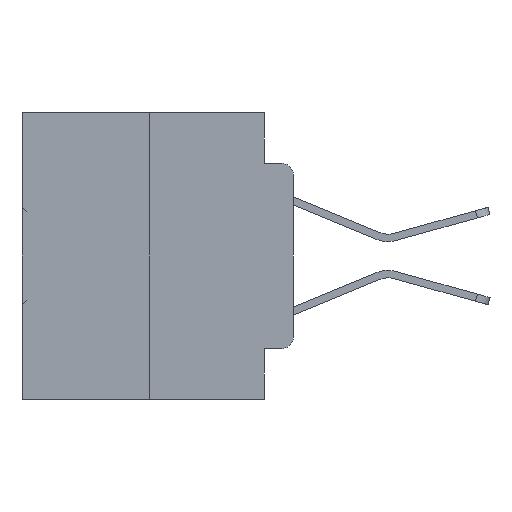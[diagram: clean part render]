
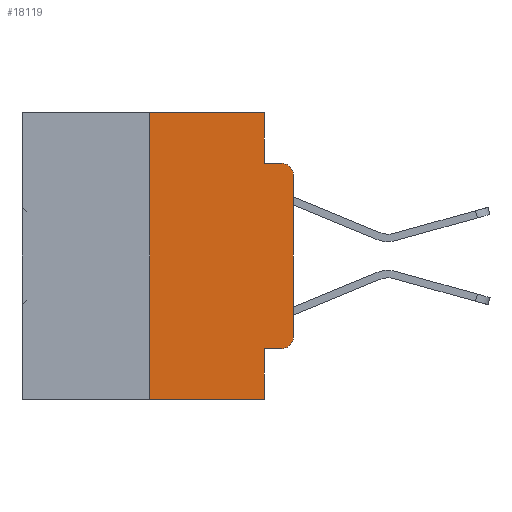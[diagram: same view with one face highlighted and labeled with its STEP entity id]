
A CAD part, left-side view. The second image highlights one B-rep face of the part: STEP entity #18119.
In plain terms, the highlighted planar face has unit normal (-1, 0, 0).
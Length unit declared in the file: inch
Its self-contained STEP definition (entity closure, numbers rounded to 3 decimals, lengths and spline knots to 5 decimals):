
#815 = CARTESIAN_POINT ( 'NONE',  ( 0., 0.02, -0.1085 ) ) ;
#1361 = VECTOR ( 'NONE', #24522, 39.37008 ) ;
#1391 = VERTEX_POINT ( 'NONE', #7197 ) ;
#2439 = VECTOR ( 'NONE', #12109, 39.37008 ) ;
#3083 = CARTESIAN_POINT ( 'NONE',  ( 0., 0.473, 0. ) ) ;
#3580 = DIRECTION ( 'NONE',  ( -1., 0., 0. ) ) ;
#4086 = CARTESIAN_POINT ( 'NONE',  ( 0., 0.02, -0.4115 ) ) ;
#4298 = DIRECTION ( 'NONE',  ( 0., 0., -1. ) ) ;
#4858 = ORIENTED_EDGE ( 'NONE', *, *, #23717, .F. ) ;
#5162 = VECTOR ( 'NONE', #30448, 39.37008 ) ;
#5226 = EDGE_CURVE ( 'NONE', #23776, #33122, #32588, .T. ) ;
#5251 = DIRECTION ( 'NONE',  ( 0., 0., -1. ) ) ;
#5301 = CARTESIAN_POINT ( 'NONE',  ( 0., 0.473, 0. ) ) ;
#6832 = CARTESIAN_POINT ( 'NONE',  ( 0., 0., -0.1085 ) ) ;
#7024 = CARTESIAN_POINT ( 'NONE',  ( 0., 0.051, 0. ) ) ;
#7197 = CARTESIAN_POINT ( 'NONE',  ( 0., 0.02, -0.0885 ) ) ;
#7627 = VERTEX_POINT ( 'NONE', #16283 ) ;
#8109 = VECTOR ( 'NONE', #4298, 39.37008 ) ;
#8132 = LINE ( 'NONE', #9540, #15769 ) ;
#8740 = DIRECTION ( 'NONE',  ( 0., 0., -1. ) ) ;
#9258 = FACE_OUTER_BOUND ( 'NONE', #24429, .T. ) ;
#9540 = CARTESIAN_POINT ( 'NONE',  ( 0., 0.051, -0.0885 ) ) ;
#9782 = CARTESIAN_POINT ( 'NONE',  ( 0., 0.051, -0.0885 ) ) ;
#9805 = VERTEX_POINT ( 'NONE', #14158 ) ;
#10071 = VECTOR ( 'NONE', #30102, 39.37008 ) ;
#10455 = LINE ( 'NONE', #14691, #2439 ) ;
#11092 = CARTESIAN_POINT ( 'NONE',  ( 0., 0.051, -0.4115 ) ) ;
#11352 = EDGE_CURVE ( 'NONE', #15332, #1391, #22079, .T. ) ;
#11834 = LINE ( 'NONE', #3083, #5162 ) ;
#12075 = CARTESIAN_POINT ( 'NONE',  ( 0., 0., 0. ) ) ;
#12109 = DIRECTION ( 'NONE',  ( 0., 0., 1. ) ) ;
#12457 = LINE ( 'NONE', #7024, #23057 ) ;
#13228 = ORIENTED_EDGE ( 'NONE', *, *, #14233, .F. ) ;
#13718 = EDGE_CURVE ( 'NONE', #17415, #15332, #17701, .T. ) ;
#13754 = AXIS2_PLACEMENT_3D ( 'NONE', #26885, #19179, #5251 ) ;
#14158 = CARTESIAN_POINT ( 'NONE',  ( 0., 0.051, -0.5 ) ) ;
#14233 = EDGE_CURVE ( 'NONE', #23814, #7627, #10455, .T. ) ;
#14691 = CARTESIAN_POINT ( 'NONE',  ( 0., 0.25, 0. ) ) ;
#15332 = VERTEX_POINT ( 'NONE', #6832 ) ;
#15384 = AXIS2_PLACEMENT_3D ( 'NONE', #5301, #26608, #24231 ) ;
#15484 = ORIENTED_EDGE ( 'NONE', *, *, #24809, .F. ) ;
#15769 = VECTOR ( 'NONE', #31266, 39.37008 ) ;
#15909 = PLANE ( 'NONE',  #15384 ) ;
#16283 = CARTESIAN_POINT ( 'NONE',  ( 0., 0.25, 0. ) ) ;
#16669 = EDGE_CURVE ( 'NONE', #22146, #18625, #17399, .T. ) ;
#17399 = LINE ( 'NONE', #33327, #8109 ) ;
#17415 = VERTEX_POINT ( 'NONE', #24233 ) ;
#17701 = LINE ( 'NONE', #12075, #18967 ) ;
#18119 = ADVANCED_FACE ( 'NONE', ( #9258 ), #15909, .F. ) ;
#18625 = VERTEX_POINT ( 'NONE', #9782 ) ;
#18967 = VECTOR ( 'NONE', #34099, 39.37008 ) ;
#19179 = DIRECTION ( 'NONE',  ( -1., 0., 0. ) ) ;
#20982 = DIRECTION ( 'NONE',  ( 0., 0., -1. ) ) ;
#21696 = ORIENTED_EDGE ( 'NONE', *, *, #13718, .T. ) ;
#22061 = ORIENTED_EDGE ( 'NONE', *, *, #5226, .T. ) ;
#22079 = CIRCLE ( 'NONE', #35113, 0.02 ) ;
#22146 = VERTEX_POINT ( 'NONE', #26812 ) ;
#22573 = EDGE_CURVE ( 'NONE', #23776, #9805, #12457, .T. ) ;
#22781 = CARTESIAN_POINT ( 'NONE',  ( 0., 0.25, -0.5 ) ) ;
#23057 = VECTOR ( 'NONE', #20982, 39.37008 ) ;
#23717 = EDGE_CURVE ( 'NONE', #18625, #1391, #8132, .T. ) ;
#23776 = VERTEX_POINT ( 'NONE', #33778 ) ;
#23814 = VERTEX_POINT ( 'NONE', #22781 ) ;
#24160 = EDGE_CURVE ( 'NONE', #23814, #9805, #25488, .T. ) ;
#24231 = DIRECTION ( 'NONE',  ( 0., 0., -1. ) ) ;
#24233 = CARTESIAN_POINT ( 'NONE',  ( 0., 0., -0.3915 ) ) ;
#24429 = EDGE_LOOP ( 'NONE', ( #21696, #26432, #4858, #33226, #15484, #13228, #32998, #26141, #22061, #33132 ) ) ;
#24522 = DIRECTION ( 'NONE',  ( 0., -1., 0. ) ) ;
#24809 = EDGE_CURVE ( 'NONE', #7627, #22146, #11834, .T. ) ;
#25488 = LINE ( 'NONE', #30372, #1361 ) ;
#26141 = ORIENTED_EDGE ( 'NONE', *, *, #22573, .F. ) ;
#26432 = ORIENTED_EDGE ( 'NONE', *, *, #11352, .T. ) ;
#26608 = DIRECTION ( 'NONE',  ( 1., 0., 0. ) ) ;
#26812 = CARTESIAN_POINT ( 'NONE',  ( 0., 0.051, 0. ) ) ;
#26885 = CARTESIAN_POINT ( 'NONE',  ( 0., 0.02, -0.3915 ) ) ;
#30102 = DIRECTION ( 'NONE',  ( 0., -1., 0. ) ) ;
#30372 = CARTESIAN_POINT ( 'NONE',  ( 0., 0.473, -0.5 ) ) ;
#30448 = DIRECTION ( 'NONE',  ( 0., -1., 0. ) ) ;
#31266 = DIRECTION ( 'NONE',  ( 0., -1., 0. ) ) ;
#31578 = EDGE_CURVE ( 'NONE', #33122, #17415, #32935, .T. ) ;
#32588 = LINE ( 'NONE', #11092, #10071 ) ;
#32935 = CIRCLE ( 'NONE', #13754, 0.02 ) ;
#32998 = ORIENTED_EDGE ( 'NONE', *, *, #24160, .T. ) ;
#33122 = VERTEX_POINT ( 'NONE', #4086 ) ;
#33132 = ORIENTED_EDGE ( 'NONE', *, *, #31578, .T. ) ;
#33226 = ORIENTED_EDGE ( 'NONE', *, *, #16669, .F. ) ;
#33327 = CARTESIAN_POINT ( 'NONE',  ( 0., 0.051, 0. ) ) ;
#33778 = CARTESIAN_POINT ( 'NONE',  ( 0., 0.051, -0.4115 ) ) ;
#34099 = DIRECTION ( 'NONE',  ( 0., 0., 1. ) ) ;
#35113 = AXIS2_PLACEMENT_3D ( 'NONE', #815, #3580, #8740 ) ;
